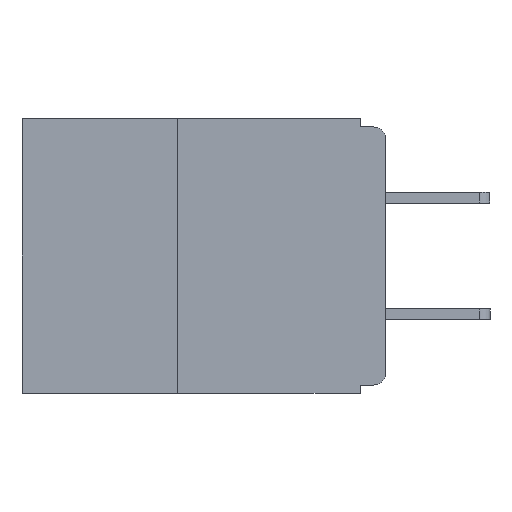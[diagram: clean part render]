
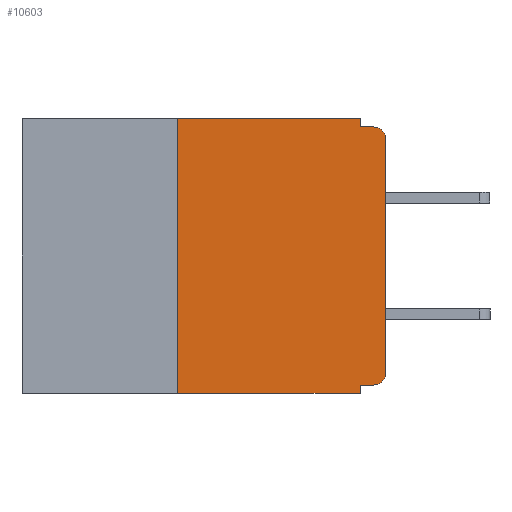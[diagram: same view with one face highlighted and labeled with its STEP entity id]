
A CAD part, left-side view. The second image highlights one B-rep face of the part: STEP entity #10603.
In plain terms, the highlighted planar face has unit normal (-1, 0, 0).
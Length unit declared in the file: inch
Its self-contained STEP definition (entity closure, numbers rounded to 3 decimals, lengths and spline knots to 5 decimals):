
#217 = ORIENTED_EDGE ( 'NONE', *, *, #718, .T. ) ;
#375 = CARTESIAN_POINT ( 'NONE',  ( 0., 0.031, 0. ) ) ;
#391 = CARTESIAN_POINT ( 'NONE',  ( 0., 0.25, -0.33 ) ) ;
#472 = AXIS2_PLACEMENT_3D ( 'NONE', #3717, #14493, #32605 ) ;
#718 = EDGE_CURVE ( 'NONE', #31954, #17305, #15343, .T. ) ;
#836 = EDGE_CURVE ( 'NONE', #31581, #31954, #16558, .T. ) ;
#2073 = DIRECTION ( 'NONE',  ( 0., 0., -1. ) ) ;
#2316 = CARTESIAN_POINT ( 'NONE',  ( 0., 0.031, -0.33 ) ) ;
#2429 = VERTEX_POINT ( 'NONE', #22991 ) ;
#2848 = CIRCLE ( 'NONE', #5188, 0.015 ) ;
#2969 = FACE_OUTER_BOUND ( 'NONE', #8744, .T. ) ;
#3074 = CARTESIAN_POINT ( 'NONE',  ( 0., 0.031, 0. ) ) ;
#3276 = VERTEX_POINT ( 'NONE', #30514 ) ;
#3395 = DIRECTION ( 'NONE',  ( 0., 0., -1. ) ) ;
#3459 = VECTOR ( 'NONE', #29671, 39.37008 ) ;
#3473 = CARTESIAN_POINT ( 'NONE',  ( 0., 0.015, -0.32 ) ) ;
#3717 = CARTESIAN_POINT ( 'NONE',  ( 0., 0.437, 0. ) ) ;
#3830 = LINE ( 'NONE', #29925, #23432 ) ;
#3947 = EDGE_CURVE ( 'NONE', #13713, #4159, #6332, .T. ) ;
#4159 = VERTEX_POINT ( 'NONE', #24694 ) ;
#5188 = AXIS2_PLACEMENT_3D ( 'NONE', #22341, #22230, #22038 ) ;
#6051 = EDGE_CURVE ( 'NONE', #17305, #3276, #2848, .T. ) ;
#6332 = LINE ( 'NONE', #2316, #28164 ) ;
#6401 = EDGE_CURVE ( 'NONE', #14563, #4159, #19628, .T. ) ;
#6560 = VECTOR ( 'NONE', #29695, 39.37008 ) ;
#7853 = EDGE_CURVE ( 'NONE', #28374, #24824, #9043, .T. ) ;
#8193 = VECTOR ( 'NONE', #3395, 39.37008 ) ;
#8405 = CARTESIAN_POINT ( 'NONE',  ( 0., 0.437, 0. ) ) ;
#8744 = EDGE_LOOP ( 'NONE', ( #217, #25185, #24610, #10882, #17569, #10718, #33512, #31474, #24505, #15665 ) ) ;
#8927 = DIRECTION ( 'NONE',  ( 0., 0., 1. ) ) ;
#9043 = LINE ( 'NONE', #3074, #8193 ) ;
#9124 = PLANE ( 'NONE',  #472 ) ;
#10603 = ADVANCED_FACE ( 'NONE', ( #2969 ), #9124, .F. ) ;
#10636 = LINE ( 'NONE', #14047, #3459 ) ;
#10718 = ORIENTED_EDGE ( 'NONE', *, *, #21777, .F. ) ;
#10882 = ORIENTED_EDGE ( 'NONE', *, *, #7853, .F. ) ;
#11481 = LINE ( 'NONE', #8405, #23916 ) ;
#12497 = VECTOR ( 'NONE', #12838, 39.37008 ) ;
#12838 = DIRECTION ( 'NONE',  ( 0., -1., 0. ) ) ;
#13258 = EDGE_CURVE ( 'NONE', #24824, #3276, #10636, .T. ) ;
#13293 = CARTESIAN_POINT ( 'NONE',  ( 0., 0.437, -0.33 ) ) ;
#13713 = VERTEX_POINT ( 'NONE', #21740 ) ;
#14047 = CARTESIAN_POINT ( 'NONE',  ( 0., 0., -0.01 ) ) ;
#14493 = DIRECTION ( 'NONE',  ( 1., 0., 0. ) ) ;
#14563 = VERTEX_POINT ( 'NONE', #391 ) ;
#15343 = LINE ( 'NONE', #33324, #6560 ) ;
#15665 = ORIENTED_EDGE ( 'NONE', *, *, #836, .T. ) ;
#16558 = CIRCLE ( 'NONE', #16773, 0.015 ) ;
#16773 = AXIS2_PLACEMENT_3D ( 'NONE', #18095, #18600, #18246 ) ;
#17305 = VERTEX_POINT ( 'NONE', #23230 ) ;
#17569 = ORIENTED_EDGE ( 'NONE', *, *, #30247, .F. ) ;
#17980 = LINE ( 'NONE', #20689, #30072 ) ;
#18016 = DIRECTION ( 'NONE',  ( 0., 1., 0. ) ) ;
#18095 = CARTESIAN_POINT ( 'NONE',  ( 0., 0.015, -0.305 ) ) ;
#18246 = DIRECTION ( 'NONE',  ( 0., 0., -1. ) ) ;
#18600 = DIRECTION ( 'NONE',  ( -1., 0., 0. ) ) ;
#19628 = LINE ( 'NONE', #13293, #12497 ) ;
#20689 = CARTESIAN_POINT ( 'NONE',  ( 0., 0., -0.32 ) ) ;
#21740 = CARTESIAN_POINT ( 'NONE',  ( 0., 0.031, -0.32 ) ) ;
#21777 = EDGE_CURVE ( 'NONE', #14563, #2429, #3830, .T. ) ;
#22038 = DIRECTION ( 'NONE',  ( 0., 0., -1. ) ) ;
#22230 = DIRECTION ( 'NONE',  ( -1., 0., 0. ) ) ;
#22341 = CARTESIAN_POINT ( 'NONE',  ( 0., 0.015, -0.025 ) ) ;
#22991 = CARTESIAN_POINT ( 'NONE',  ( 0., 0.25, 0. ) ) ;
#23230 = CARTESIAN_POINT ( 'NONE',  ( 0., 0., -0.025 ) ) ;
#23432 = VECTOR ( 'NONE', #8927, 39.37008 ) ;
#23916 = VECTOR ( 'NONE', #29428, 39.37008 ) ;
#24505 = ORIENTED_EDGE ( 'NONE', *, *, #33625, .F. ) ;
#24610 = ORIENTED_EDGE ( 'NONE', *, *, #13258, .F. ) ;
#24694 = CARTESIAN_POINT ( 'NONE',  ( 0., 0.031, -0.33 ) ) ;
#24824 = VERTEX_POINT ( 'NONE', #27359 ) ;
#25185 = ORIENTED_EDGE ( 'NONE', *, *, #6051, .T. ) ;
#27359 = CARTESIAN_POINT ( 'NONE',  ( 0., 0.031, -0.01 ) ) ;
#28164 = VECTOR ( 'NONE', #2073, 39.37008 ) ;
#28374 = VERTEX_POINT ( 'NONE', #375 ) ;
#28647 = CARTESIAN_POINT ( 'NONE',  ( 0., 0., -0.305 ) ) ;
#29428 = DIRECTION ( 'NONE',  ( 0., -1., 0. ) ) ;
#29671 = DIRECTION ( 'NONE',  ( 0., -1., 0. ) ) ;
#29695 = DIRECTION ( 'NONE',  ( 0., 0., 1. ) ) ;
#29925 = CARTESIAN_POINT ( 'NONE',  ( 0., 0.25, -0.33 ) ) ;
#30072 = VECTOR ( 'NONE', #18016, 39.37008 ) ;
#30247 = EDGE_CURVE ( 'NONE', #2429, #28374, #11481, .T. ) ;
#30514 = CARTESIAN_POINT ( 'NONE',  ( 0., 0.015, -0.01 ) ) ;
#31474 = ORIENTED_EDGE ( 'NONE', *, *, #3947, .F. ) ;
#31581 = VERTEX_POINT ( 'NONE', #3473 ) ;
#31954 = VERTEX_POINT ( 'NONE', #28647 ) ;
#32605 = DIRECTION ( 'NONE',  ( 0., 0., -1. ) ) ;
#33324 = CARTESIAN_POINT ( 'NONE',  ( 0., 0., 0. ) ) ;
#33512 = ORIENTED_EDGE ( 'NONE', *, *, #6401, .T. ) ;
#33625 = EDGE_CURVE ( 'NONE', #31581, #13713, #17980, .T. ) ;
